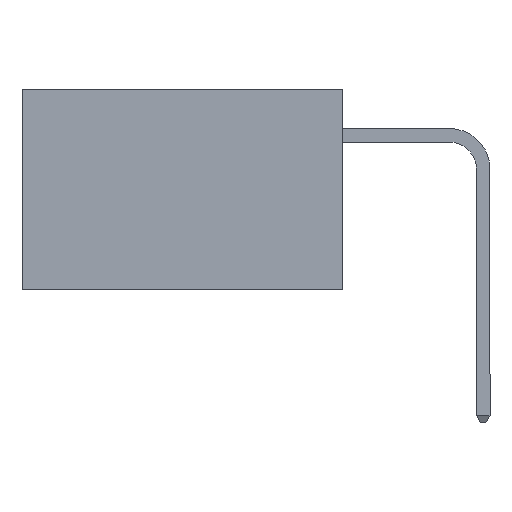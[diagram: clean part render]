
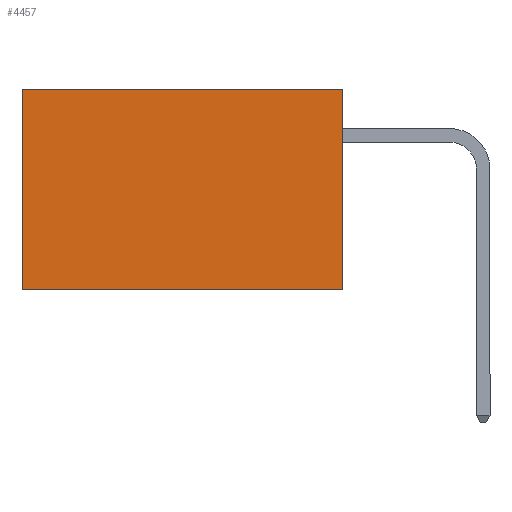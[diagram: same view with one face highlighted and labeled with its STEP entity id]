
A CAD part, left-side view. The second image highlights one B-rep face of the part: STEP entity #4457.
In plain terms, the highlighted planar face has unit normal (-1, 0, 0).
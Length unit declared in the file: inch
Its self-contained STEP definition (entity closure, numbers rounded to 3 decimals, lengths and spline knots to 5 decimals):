
#345 = AXIS2_PLACEMENT_3D ( 'NONE', #10820, #6742, #6711 ) ;
#416 = VERTEX_POINT ( 'NONE', #9493 ) ;
#1007 = DIRECTION ( 'NONE',  ( 0., 1., 0. ) ) ;
#1246 = VECTOR ( 'NONE', #4205, 39.37008 ) ;
#2432 = EDGE_LOOP ( 'NONE', ( #4275, #2920, #2795, #2759 ) ) ;
#2759 = ORIENTED_EDGE ( 'NONE', *, *, #8921, .T. ) ;
#2795 = ORIENTED_EDGE ( 'NONE', *, *, #7742, .F. ) ;
#2920 = ORIENTED_EDGE ( 'NONE', *, *, #9714, .F. ) ;
#3084 = LINE ( 'NONE', #9689, #4905 ) ;
#4205 = DIRECTION ( 'NONE',  ( 0., 1., 0. ) ) ;
#4275 = ORIENTED_EDGE ( 'NONE', *, *, #8848, .T. ) ;
#4353 = VECTOR ( 'NONE', #1007, 39.37008 ) ;
#4457 = ADVANCED_FACE ( 'NONE', ( #5097 ), #9854, .F. ) ;
#4905 = VECTOR ( 'NONE', #8081, 39.37008 ) ;
#5097 = FACE_OUTER_BOUND ( 'NONE', #2432, .T. ) ;
#5225 = CARTESIAN_POINT ( 'NONE',  ( 0.277, 0.59, 0. ) ) ;
#5455 = CARTESIAN_POINT ( 'NONE',  ( 0.277, 0.59, -0.37 ) ) ;
#6051 = CARTESIAN_POINT ( 'NONE',  ( 0.277, 0., 0. ) ) ;
#6711 = DIRECTION ( 'NONE',  ( 0., 0., -1. ) ) ;
#6742 = DIRECTION ( 'NONE',  ( 1., 0., 0. ) ) ;
#6890 = LINE ( 'NONE', #7298, #4353 ) ;
#7298 = CARTESIAN_POINT ( 'NONE',  ( 0.277, 0., 0. ) ) ;
#7671 = LINE ( 'NONE', #5455, #9578 ) ;
#7717 = CARTESIAN_POINT ( 'NONE',  ( 0.277, 0., -0.37 ) ) ;
#7742 = EDGE_CURVE ( 'NONE', #8652, #10463, #3084, .T. ) ;
#8081 = DIRECTION ( 'NONE',  ( 0., 0., -1. ) ) ;
#8652 = VERTEX_POINT ( 'NONE', #6051 ) ;
#8674 = VERTEX_POINT ( 'NONE', #5225 ) ;
#8848 = EDGE_CURVE ( 'NONE', #8674, #416, #7671, .T. ) ;
#8921 = EDGE_CURVE ( 'NONE', #8652, #8674, #6890, .T. ) ;
#9493 = CARTESIAN_POINT ( 'NONE',  ( 0.277, 0.59, -0.37 ) ) ;
#9578 = VECTOR ( 'NONE', #10430, 39.37008 ) ;
#9689 = CARTESIAN_POINT ( 'NONE',  ( 0.277, 0., -0.37 ) ) ;
#9714 = EDGE_CURVE ( 'NONE', #10463, #416, #10469, .T. ) ;
#9854 = PLANE ( 'NONE',  #345 ) ;
#10051 = CARTESIAN_POINT ( 'NONE',  ( 0.277, 0., -0.37 ) ) ;
#10430 = DIRECTION ( 'NONE',  ( 0., 0., -1. ) ) ;
#10463 = VERTEX_POINT ( 'NONE', #7717 ) ;
#10469 = LINE ( 'NONE', #10051, #1246 ) ;
#10820 = CARTESIAN_POINT ( 'NONE',  ( 0.277, 0., -0.37 ) ) ;
